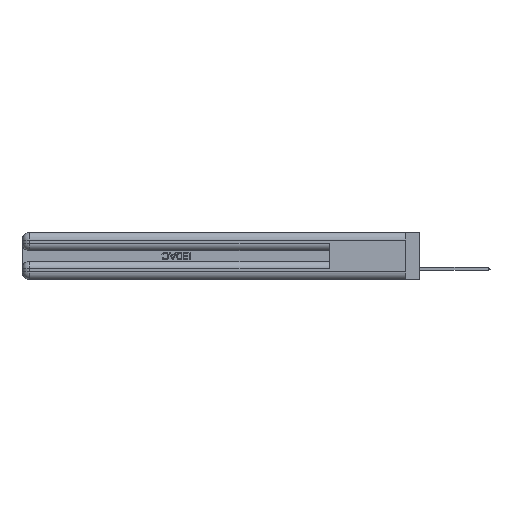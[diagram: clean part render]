
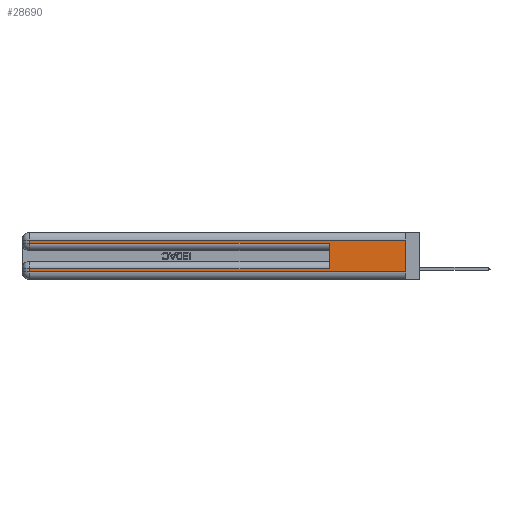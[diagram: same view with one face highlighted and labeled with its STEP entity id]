
A CAD part, left-side view. The second image highlights one B-rep face of the part: STEP entity #28690.
In plain terms, the highlighted planar face has unit normal (-1, 0, 0).
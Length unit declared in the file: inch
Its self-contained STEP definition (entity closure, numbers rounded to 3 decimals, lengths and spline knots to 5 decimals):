
#693 = DIRECTION ( 'NONE',  ( 1., 0., 0. ) ) ;
#1784 = CARTESIAN_POINT ( 'NONE',  ( 0., 0.6, 0.085 ) ) ;
#2600 = CARTESIAN_POINT ( 'NONE',  ( 0., 0., 0.06 ) ) ;
#3524 = VERTEX_POINT ( 'NONE', #47653 ) ;
#4039 = EDGE_CURVE ( 'NONE', #40101, #24830, #26940, .T. ) ;
#4075 = DIRECTION ( 'NONE',  ( 0., -1., 0. ) ) ;
#4479 = PLANE ( 'NONE',  #40907 ) ;
#5761 = CARTESIAN_POINT ( 'NONE',  ( 0., 2.94, 0.06 ) ) ;
#5921 = CARTESIAN_POINT ( 'NONE',  ( 0., 0.6, 0.285 ) ) ;
#6671 = ORIENTED_EDGE ( 'NONE', *, *, #4039, .T. ) ;
#6902 = EDGE_CURVE ( 'NONE', #24830, #12688, #21828, .T. ) ;
#7257 = CARTESIAN_POINT ( 'NONE',  ( 0., 0., 0.085 ) ) ;
#7377 = CARTESIAN_POINT ( 'NONE',  ( 0., 2.94, 0.31 ) ) ;
#7443 = DIRECTION ( 'NONE',  ( 0., 1., 0. ) ) ;
#7588 = DIRECTION ( 'NONE',  ( 0., 1., 0. ) ) ;
#8238 = ORIENTED_EDGE ( 'NONE', *, *, #17163, .F. ) ;
#8376 = FACE_OUTER_BOUND ( 'NONE', #17906, .T. ) ;
#8499 = ORIENTED_EDGE ( 'NONE', *, *, #6902, .T. ) ;
#10831 = EDGE_CURVE ( 'NONE', #40101, #15171, #43038, .T. ) ;
#11728 = ORIENTED_EDGE ( 'NONE', *, *, #48114, .T. ) ;
#12688 = VERTEX_POINT ( 'NONE', #5761 ) ;
#13867 = DIRECTION ( 'NONE',  ( 0., 0., -1. ) ) ;
#15171 = VERTEX_POINT ( 'NONE', #5921 ) ;
#15474 = VECTOR ( 'NONE', #22706, 39.37008 ) ;
#17163 = EDGE_CURVE ( 'NONE', #3524, #44717, #37201, .T. ) ;
#17906 = EDGE_LOOP ( 'NONE', ( #8238, #19003, #20068, #11728, #35291, #6671, #8499, #18951 ) ) ;
#18030 = CARTESIAN_POINT ( 'NONE',  ( 0., 0.6, 0.145 ) ) ;
#18375 = DIRECTION ( 'NONE',  ( 0., 0., 1. ) ) ;
#18843 = CARTESIAN_POINT ( 'NONE',  ( 0., 2.94, 0.085 ) ) ;
#18951 = ORIENTED_EDGE ( 'NONE', *, *, #35976, .T. ) ;
#19003 = ORIENTED_EDGE ( 'NONE', *, *, #22411, .T. ) ;
#20068 = ORIENTED_EDGE ( 'NONE', *, *, #49683, .T. ) ;
#21828 = LINE ( 'NONE', #44537, #41087 ) ;
#22411 = EDGE_CURVE ( 'NONE', #3524, #24285, #23947, .T. ) ;
#22706 = DIRECTION ( 'NONE',  ( 0., 0., -1. ) ) ;
#23773 = LINE ( 'NONE', #24443, #30442 ) ;
#23947 = LINE ( 'NONE', #42877, #33014 ) ;
#24285 = VERTEX_POINT ( 'NONE', #7377 ) ;
#24443 = CARTESIAN_POINT ( 'NONE',  ( 0., 0., 0.06 ) ) ;
#24830 = VERTEX_POINT ( 'NONE', #18843 ) ;
#26784 = CARTESIAN_POINT ( 'NONE',  ( 0., 2.94, 0.285 ) ) ;
#26940 = LINE ( 'NONE', #7257, #39520 ) ;
#27476 = DIRECTION ( 'NONE',  ( 0., 0., -1. ) ) ;
#27537 = VECTOR ( 'NONE', #39724, 39.37008 ) ;
#28690 = ADVANCED_FACE ( 'NONE', ( #8376 ), #4479, .F. ) ;
#30442 = VECTOR ( 'NONE', #36413, 39.37008 ) ;
#31056 = VECTOR ( 'NONE', #4075, 39.37008 ) ;
#31538 = CARTESIAN_POINT ( 'NONE',  ( 0., 0., 0.285 ) ) ;
#31638 = CARTESIAN_POINT ( 'NONE',  ( 0., 0., 0.37 ) ) ;
#32220 = LINE ( 'NONE', #31538, #31056 ) ;
#32811 = VECTOR ( 'NONE', #18375, 39.37008 ) ;
#33014 = VECTOR ( 'NONE', #7443, 39.37008 ) ;
#35291 = ORIENTED_EDGE ( 'NONE', *, *, #10831, .F. ) ;
#35976 = EDGE_CURVE ( 'NONE', #12688, #44717, #23773, .T. ) ;
#36413 = DIRECTION ( 'NONE',  ( 0., -1., 0. ) ) ;
#37201 = LINE ( 'NONE', #40418, #27537 ) ;
#38214 = CARTESIAN_POINT ( 'NONE',  ( 0., 2.94, 0.37 ) ) ;
#39520 = VECTOR ( 'NONE', #7588, 39.37008 ) ;
#39571 = LINE ( 'NONE', #38214, #15474 ) ;
#39724 = DIRECTION ( 'NONE',  ( 0., 0., -1. ) ) ;
#40101 = VERTEX_POINT ( 'NONE', #1784 ) ;
#40418 = CARTESIAN_POINT ( 'NONE',  ( 0., 0., 0.37 ) ) ;
#40907 = AXIS2_PLACEMENT_3D ( 'NONE', #31638, #693, #27476 ) ;
#41087 = VECTOR ( 'NONE', #13867, 39.37008 ) ;
#42877 = CARTESIAN_POINT ( 'NONE',  ( 0., 0., 0.31 ) ) ;
#43038 = LINE ( 'NONE', #18030, #32811 ) ;
#44537 = CARTESIAN_POINT ( 'NONE',  ( 0., 2.94, 0.37 ) ) ;
#44717 = VERTEX_POINT ( 'NONE', #2600 ) ;
#46628 = VERTEX_POINT ( 'NONE', #26784 ) ;
#47653 = CARTESIAN_POINT ( 'NONE',  ( 0., 0., 0.31 ) ) ;
#48114 = EDGE_CURVE ( 'NONE', #46628, #15171, #32220, .T. ) ;
#49683 = EDGE_CURVE ( 'NONE', #24285, #46628, #39571, .T. ) ;
